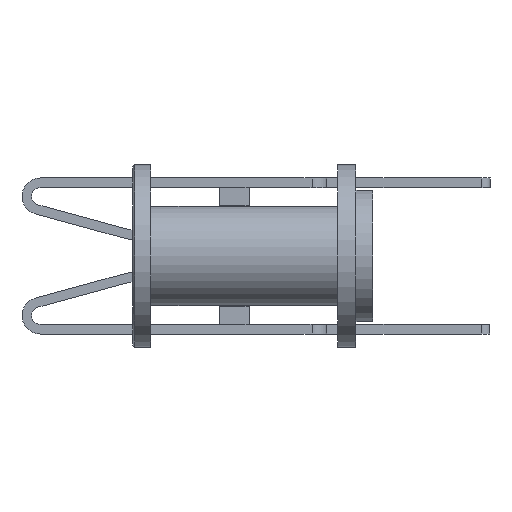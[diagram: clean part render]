
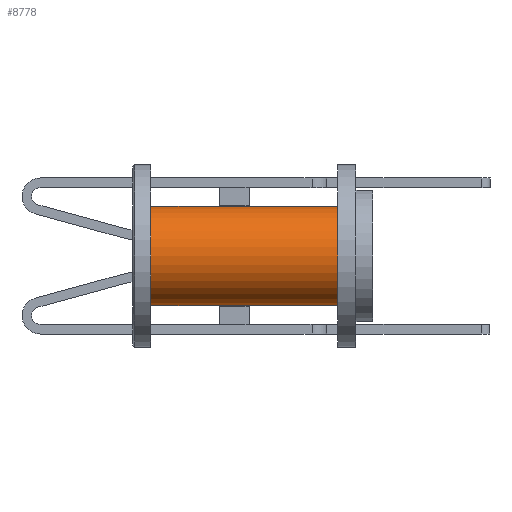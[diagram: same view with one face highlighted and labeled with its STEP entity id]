
A CAD part, left-side view. The second image highlights one B-rep face of the part: STEP entity #8778.
In plain terms, the highlighted cylindrical face has radius 1.727 mm (diameter 3.454 mm), a partial arc.
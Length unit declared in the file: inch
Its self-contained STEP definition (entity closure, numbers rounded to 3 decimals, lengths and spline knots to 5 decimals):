
#260 = CARTESIAN_POINT ( 'NONE',  ( 0., 0.28, 0. ) ) ;
#678 = CYLINDRICAL_SURFACE ( 'NONE', #14680, 0.068 ) ;
#1279 = FACE_OUTER_BOUND ( 'NONE', #8075, .T. ) ;
#2175 = DIRECTION ( 'NONE',  ( 0., 0., 1. ) ) ;
#2776 = EDGE_CURVE ( 'NONE', #21459, #11095, #10708, .T. ) ;
#2979 = EDGE_CURVE ( 'NONE', #21459, #13062, #20341, .T. ) ;
#2985 = CARTESIAN_POINT ( 'NONE',  ( 0., 0.328, 0. ) ) ;
#3579 = CARTESIAN_POINT ( 'NONE',  ( 0., 0.28, -0.068 ) ) ;
#4793 = DIRECTION ( 'NONE',  ( 0., -1., 0. ) ) ;
#5380 = DIRECTION ( 'NONE',  ( 0., 1., 0. ) ) ;
#5474 = ORIENTED_EDGE ( 'NONE', *, *, #2776, .F. ) ;
#5754 = ORIENTED_EDGE ( 'NONE', *, *, #2979, .T. ) ;
#8075 = EDGE_LOOP ( 'NONE', ( #17006, #5474, #5754, #8407 ) ) ;
#8407 = ORIENTED_EDGE ( 'NONE', *, *, #9745, .T. ) ;
#8461 = VECTOR ( 'NONE', #14109, 39.37008 ) ;
#8599 = CARTESIAN_POINT ( 'NONE',  ( 0., 0.28, 0.068 ) ) ;
#8778 = ADVANCED_FACE ( 'NONE', ( #1279 ), #678, .T. ) ;
#8824 = AXIS2_PLACEMENT_3D ( 'NONE', #260, #12691, #2175 ) ;
#9745 = EDGE_CURVE ( 'NONE', #13062, #18764, #16047, .T. ) ;
#10708 = CIRCLE ( 'NONE', #8824, 0.068 ) ;
#11007 = CARTESIAN_POINT ( 'NONE',  ( 0., 0.025, -0.068 ) ) ;
#11095 = VERTEX_POINT ( 'NONE', #8599 ) ;
#11212 = EDGE_CURVE ( 'NONE', #11095, #18764, #17567, .T. ) ;
#12691 = DIRECTION ( 'NONE',  ( 0., 1., 0. ) ) ;
#13062 = VERTEX_POINT ( 'NONE', #11007 ) ;
#14109 = DIRECTION ( 'NONE',  ( 0., -1., 0. ) ) ;
#14680 = AXIS2_PLACEMENT_3D ( 'NONE', #2985, #4793, #16839 ) ;
#14832 = CARTESIAN_POINT ( 'NONE',  ( 0., 0.328, -0.068 ) ) ;
#14984 = AXIS2_PLACEMENT_3D ( 'NONE', #15714, #5380, #17401 ) ;
#15474 = VECTOR ( 'NONE', #18189, 39.37008 ) ;
#15714 = CARTESIAN_POINT ( 'NONE',  ( 0., 0.025, 0. ) ) ;
#15976 = CARTESIAN_POINT ( 'NONE',  ( 0., 0.025, 0.068 ) ) ;
#16047 = CIRCLE ( 'NONE', #14984, 0.068 ) ;
#16839 = DIRECTION ( 'NONE',  ( 0., 0., -1. ) ) ;
#17006 = ORIENTED_EDGE ( 'NONE', *, *, #11212, .F. ) ;
#17401 = DIRECTION ( 'NONE',  ( 0., 0., 1. ) ) ;
#17567 = LINE ( 'NONE', #22284, #8461 ) ;
#18189 = DIRECTION ( 'NONE',  ( 0., -1., 0. ) ) ;
#18764 = VERTEX_POINT ( 'NONE', #15976 ) ;
#20341 = LINE ( 'NONE', #14832, #15474 ) ;
#21459 = VERTEX_POINT ( 'NONE', #3579 ) ;
#22284 = CARTESIAN_POINT ( 'NONE',  ( 0., 0.328, 0.068 ) ) ;
